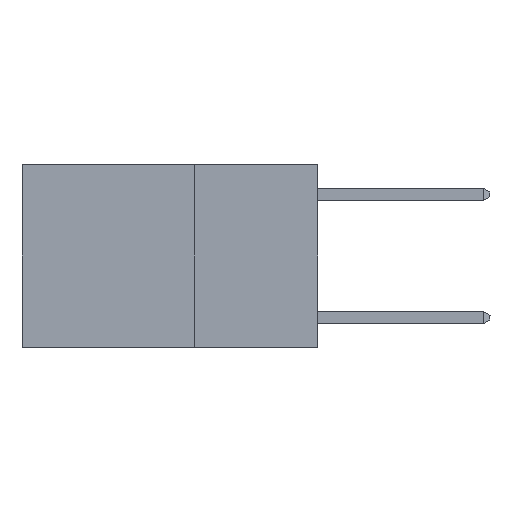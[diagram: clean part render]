
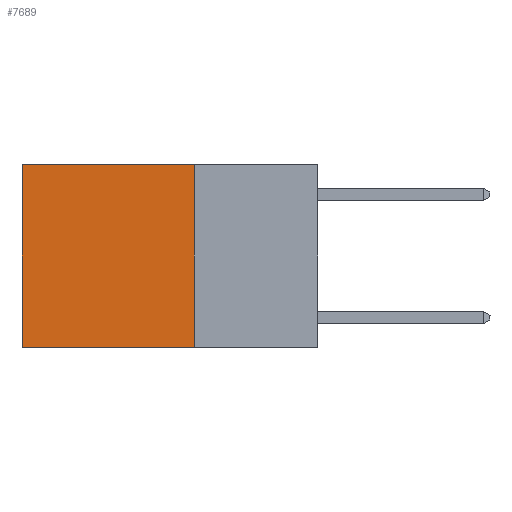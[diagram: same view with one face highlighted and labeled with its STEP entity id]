
A CAD part, left-side view. The second image highlights one B-rep face of the part: STEP entity #7689.
In plain terms, the highlighted planar face has unit normal (-1, 0, 0).
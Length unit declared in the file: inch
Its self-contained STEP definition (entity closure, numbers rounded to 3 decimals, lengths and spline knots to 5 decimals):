
#172 = VERTEX_POINT ( 'NONE', #13569 ) ;
#826 = PLANE ( 'NONE',  #4564 ) ;
#1114 = ORIENTED_EDGE ( 'NONE', *, *, #9996, .T. ) ;
#1119 = DIRECTION ( 'NONE',  ( 0., 1., 0. ) ) ;
#1489 = LINE ( 'NONE', #2626, #4967 ) ;
#2626 = CARTESIAN_POINT ( 'NONE',  ( 0.2625, 0.25, 0. ) ) ;
#3470 = EDGE_LOOP ( 'NONE', ( #1114, #13588, #11953, #18070 ) ) ;
#3693 = VECTOR ( 'NONE', #12758, 39.37008 ) ;
#4564 = AXIS2_PLACEMENT_3D ( 'NONE', #14387, #16078, #5992 ) ;
#4967 = VECTOR ( 'NONE', #16075, 39.37008 ) ;
#5992 = DIRECTION ( 'NONE',  ( 0., 0., -1. ) ) ;
#7689 = ADVANCED_FACE ( 'NONE', ( #7795 ), #826, .F. ) ;
#7795 = FACE_OUTER_BOUND ( 'NONE', #3470, .T. ) ;
#7893 = CARTESIAN_POINT ( 'NONE',  ( 0.2625, 0.25, 0. ) ) ;
#7978 = CARTESIAN_POINT ( 'NONE',  ( 0.2625, 0.25, 0. ) ) ;
#8234 = LINE ( 'NONE', #19452, #3693 ) ;
#9065 = EDGE_CURVE ( 'NONE', #20133, #172, #16699, .T. ) ;
#9996 = EDGE_CURVE ( 'NONE', #13418, #172, #8234, .T. ) ;
#10109 = VECTOR ( 'NONE', #1119, 39.37008 ) ;
#10627 = LINE ( 'NONE', #7893, #10109 ) ;
#11400 = CARTESIAN_POINT ( 'NONE',  ( 0.2625, 0.25, -0.37 ) ) ;
#11519 = EDGE_CURVE ( 'NONE', #11618, #20133, #1489, .T. ) ;
#11618 = VERTEX_POINT ( 'NONE', #7978 ) ;
#11953 = ORIENTED_EDGE ( 'NONE', *, *, #11519, .F. ) ;
#12758 = DIRECTION ( 'NONE',  ( 0., 0., -1. ) ) ;
#13418 = VERTEX_POINT ( 'NONE', #13952 ) ;
#13569 = CARTESIAN_POINT ( 'NONE',  ( 0.2625, 0.6, -0.37 ) ) ;
#13588 = ORIENTED_EDGE ( 'NONE', *, *, #9065, .F. ) ;
#13691 = CARTESIAN_POINT ( 'NONE',  ( 0.2625, 0.25, -0.37 ) ) ;
#13952 = CARTESIAN_POINT ( 'NONE',  ( 0.2625, 0.6, 0. ) ) ;
#14387 = CARTESIAN_POINT ( 'NONE',  ( 0.2625, 0.25, 0. ) ) ;
#15365 = DIRECTION ( 'NONE',  ( 0., 1., 0. ) ) ;
#15622 = EDGE_CURVE ( 'NONE', #11618, #13418, #10627, .T. ) ;
#16075 = DIRECTION ( 'NONE',  ( 0., 0., -1. ) ) ;
#16078 = DIRECTION ( 'NONE',  ( 1., 0., 0. ) ) ;
#16699 = LINE ( 'NONE', #13691, #17741 ) ;
#17741 = VECTOR ( 'NONE', #15365, 39.37008 ) ;
#18070 = ORIENTED_EDGE ( 'NONE', *, *, #15622, .T. ) ;
#19452 = CARTESIAN_POINT ( 'NONE',  ( 0.2625, 0.6, 0. ) ) ;
#20133 = VERTEX_POINT ( 'NONE', #11400 ) ;
